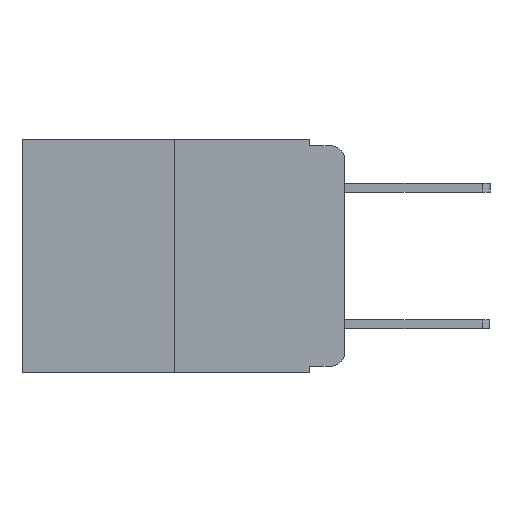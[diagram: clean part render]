
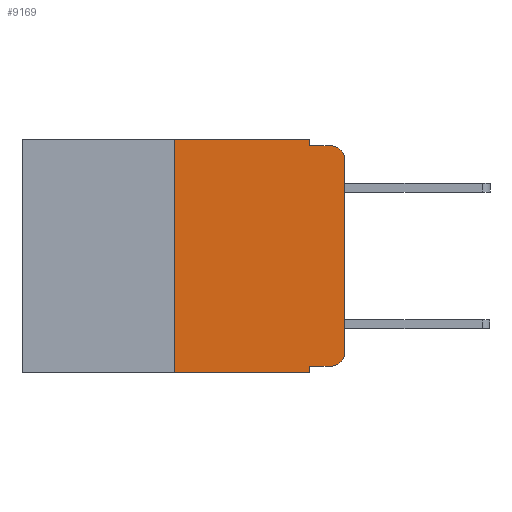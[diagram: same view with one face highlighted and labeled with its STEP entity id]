
A CAD part, left-side view. The second image highlights one B-rep face of the part: STEP entity #9169.
In plain terms, the highlighted planar face has unit normal (-1, 0, 0).
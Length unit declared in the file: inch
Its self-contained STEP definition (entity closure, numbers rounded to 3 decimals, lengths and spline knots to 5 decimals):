
#260 = VECTOR ( 'NONE', #8736, 39.37008 ) ;
#497 = VERTEX_POINT ( 'NONE', #8508 ) ;
#534 = ORIENTED_EDGE ( 'NONE', *, *, #10352, .F. ) ;
#776 = CARTESIAN_POINT ( 'NONE',  ( 0., 0., -0.313 ) ) ;
#879 = ORIENTED_EDGE ( 'NONE', *, *, #6573, .T. ) ;
#923 = DIRECTION ( 'NONE',  ( 0., -1., 0. ) ) ;
#1074 = DIRECTION ( 'NONE',  ( 0., -1., 0. ) ) ;
#1103 = CARTESIAN_POINT ( 'NONE',  ( 0., 0.25, 0. ) ) ;
#1189 = ORIENTED_EDGE ( 'NONE', *, *, #4076, .T. ) ;
#1340 = LINE ( 'NONE', #11331, #10275 ) ;
#1740 = CARTESIAN_POINT ( 'NONE',  ( 0., 0.473, 0. ) ) ;
#1771 = DIRECTION ( 'NONE',  ( 0., 0., -1. ) ) ;
#2024 = VECTOR ( 'NONE', #9817, 39.37008 ) ;
#2521 = VERTEX_POINT ( 'NONE', #10715 ) ;
#2832 = EDGE_CURVE ( 'NONE', #9117, #3355, #8664, .T. ) ;
#2864 = VERTEX_POINT ( 'NONE', #4510 ) ;
#2927 = ORIENTED_EDGE ( 'NONE', *, *, #9288, .F. ) ;
#2970 = DIRECTION ( 'NONE',  ( -1., 0., 0. ) ) ;
#3070 = VERTEX_POINT ( 'NONE', #4409 ) ;
#3355 = VERTEX_POINT ( 'NONE', #5545 ) ;
#3390 = VERTEX_POINT ( 'NONE', #8334 ) ;
#3420 = CARTESIAN_POINT ( 'NONE',  ( 0., 0.02, -0.313 ) ) ;
#3462 = FACE_OUTER_BOUND ( 'NONE', #4824, .T. ) ;
#3503 = ORIENTED_EDGE ( 'NONE', *, *, #10870, .F. ) ;
#3980 = VECTOR ( 'NONE', #1074, 39.37008 ) ;
#4001 = DIRECTION ( 'NONE',  ( 0., 0., 1. ) ) ;
#4076 = EDGE_CURVE ( 'NONE', #3355, #5459, #10139, .T. ) ;
#4409 = CARTESIAN_POINT ( 'NONE',  ( 0., 0.051, -0.343 ) ) ;
#4461 = VECTOR ( 'NONE', #923, 39.37008 ) ;
#4510 = CARTESIAN_POINT ( 'NONE',  ( 0., 0., -0.03 ) ) ;
#4777 = VECTOR ( 'NONE', #10571, 39.37008 ) ;
#4824 = EDGE_LOOP ( 'NONE', ( #5037, #7296, #2927, #5307, #9676, #534, #879, #3503, #10163, #1189 ) ) ;
#4874 = CARTESIAN_POINT ( 'NONE',  ( 0., 0.051, 0. ) ) ;
#5037 = ORIENTED_EDGE ( 'NONE', *, *, #7177, .T. ) ;
#5307 = ORIENTED_EDGE ( 'NONE', *, *, #9847, .F. ) ;
#5331 = VERTEX_POINT ( 'NONE', #8735 ) ;
#5459 = VERTEX_POINT ( 'NONE', #776 ) ;
#5545 = CARTESIAN_POINT ( 'NONE',  ( 0., 0.02, -0.333 ) ) ;
#5574 = VECTOR ( 'NONE', #10624, 39.37008 ) ;
#5585 = DIRECTION ( 'NONE',  ( 0., 0., -1. ) ) ;
#5644 = DIRECTION ( 'NONE',  ( -1., 0., 0. ) ) ;
#5858 = EDGE_CURVE ( 'NONE', #9668, #5331, #10545, .T. ) ;
#5971 = VECTOR ( 'NONE', #9030, 39.37008 ) ;
#5979 = AXIS2_PLACEMENT_3D ( 'NONE', #8114, #2970, #8899 ) ;
#6300 = CARTESIAN_POINT ( 'NONE',  ( 0., 0.473, 0. ) ) ;
#6573 = EDGE_CURVE ( 'NONE', #3390, #3070, #8063, .T. ) ;
#6640 = CARTESIAN_POINT ( 'NONE',  ( 0., 0.473, -0.343 ) ) ;
#6872 = CARTESIAN_POINT ( 'NONE',  ( 0., 0.051, -0.333 ) ) ;
#7014 = CARTESIAN_POINT ( 'NONE',  ( 0., 0.25, 0. ) ) ;
#7169 = DIRECTION ( 'NONE',  ( 1., 0., 0. ) ) ;
#7177 = EDGE_CURVE ( 'NONE', #5459, #2864, #1340, .T. ) ;
#7293 = CARTESIAN_POINT ( 'NONE',  ( 0., 0.051, -0.01 ) ) ;
#7296 = ORIENTED_EDGE ( 'NONE', *, *, #8228, .T. ) ;
#7760 = CIRCLE ( 'NONE', #5979, 0.02 ) ;
#7860 = CARTESIAN_POINT ( 'NONE',  ( 0., 0.051, -0.333 ) ) ;
#8063 = LINE ( 'NONE', #6640, #5574 ) ;
#8114 = CARTESIAN_POINT ( 'NONE',  ( 0., 0.02, -0.03 ) ) ;
#8228 = EDGE_CURVE ( 'NONE', #2864, #2521, #7760, .T. ) ;
#8287 = AXIS2_PLACEMENT_3D ( 'NONE', #3420, #5644, #5585 ) ;
#8334 = CARTESIAN_POINT ( 'NONE',  ( 0., 0.25, -0.343 ) ) ;
#8405 = LINE ( 'NONE', #1103, #5971 ) ;
#8508 = CARTESIAN_POINT ( 'NONE',  ( 0., 0.051, -0.01 ) ) ;
#8664 = LINE ( 'NONE', #6872, #2024 ) ;
#8735 = CARTESIAN_POINT ( 'NONE',  ( 0., 0.051, 0. ) ) ;
#8736 = DIRECTION ( 'NONE',  ( 0., 0., -1. ) ) ;
#8864 = LINE ( 'NONE', #7293, #4461 ) ;
#8899 = DIRECTION ( 'NONE',  ( 0., 0., -1. ) ) ;
#8907 = LINE ( 'NONE', #4874, #4777 ) ;
#9030 = DIRECTION ( 'NONE',  ( 0., 0., 1. ) ) ;
#9117 = VERTEX_POINT ( 'NONE', #7860 ) ;
#9169 = ADVANCED_FACE ( 'NONE', ( #3462 ), #11100, .F. ) ;
#9288 = EDGE_CURVE ( 'NONE', #497, #2521, #8864, .T. ) ;
#9487 = LINE ( 'NONE', #11124, #260 ) ;
#9668 = VERTEX_POINT ( 'NONE', #7014 ) ;
#9676 = ORIENTED_EDGE ( 'NONE', *, *, #5858, .F. ) ;
#9739 = AXIS2_PLACEMENT_3D ( 'NONE', #6300, #7169, #1771 ) ;
#9817 = DIRECTION ( 'NONE',  ( 0., -1., 0. ) ) ;
#9847 = EDGE_CURVE ( 'NONE', #5331, #497, #9487, .T. ) ;
#10139 = CIRCLE ( 'NONE', #8287, 0.02 ) ;
#10163 = ORIENTED_EDGE ( 'NONE', *, *, #2832, .T. ) ;
#10275 = VECTOR ( 'NONE', #4001, 39.37008 ) ;
#10352 = EDGE_CURVE ( 'NONE', #3390, #9668, #8405, .T. ) ;
#10545 = LINE ( 'NONE', #1740, #3980 ) ;
#10571 = DIRECTION ( 'NONE',  ( 0., 0., -1. ) ) ;
#10624 = DIRECTION ( 'NONE',  ( 0., -1., 0. ) ) ;
#10715 = CARTESIAN_POINT ( 'NONE',  ( 0., 0.02, -0.01 ) ) ;
#10870 = EDGE_CURVE ( 'NONE', #9117, #3070, #8907, .T. ) ;
#11100 = PLANE ( 'NONE',  #9739 ) ;
#11124 = CARTESIAN_POINT ( 'NONE',  ( 0., 0.051, 0. ) ) ;
#11331 = CARTESIAN_POINT ( 'NONE',  ( 0., 0., 0. ) ) ;
